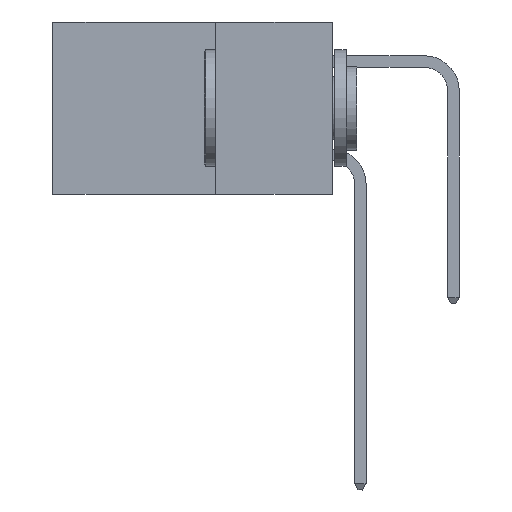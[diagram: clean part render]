
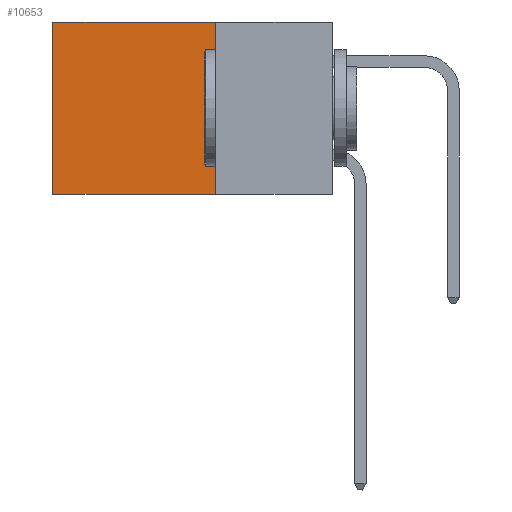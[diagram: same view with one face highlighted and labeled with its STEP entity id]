
A CAD part, left-side view. The second image highlights one B-rep face of the part: STEP entity #10653.
In plain terms, the highlighted planar face has unit normal (-1, 0, 0).
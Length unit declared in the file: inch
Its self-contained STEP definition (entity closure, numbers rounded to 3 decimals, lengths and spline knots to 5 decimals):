
#23 = DIRECTION ( 'NONE',  ( 0., 1., 0. ) ) ;
#202 = DIRECTION ( 'NONE',  ( 0., 1., 0. ) ) ;
#2963 = VERTEX_POINT ( 'NONE', #16725 ) ;
#3412 = CARTESIAN_POINT ( 'NONE',  ( 0.298, 0.25, 0. ) ) ;
#3432 = AXIS2_PLACEMENT_3D ( 'NONE', #3412, #16153, #6880 ) ;
#4799 = EDGE_LOOP ( 'NONE', ( #21293, #13506, #5982, #21306 ) ) ;
#5472 = VERTEX_POINT ( 'NONE', #6373 ) ;
#5982 = ORIENTED_EDGE ( 'NONE', *, *, #19559, .F. ) ;
#6373 = CARTESIAN_POINT ( 'NONE',  ( 0.298, 0.25, 0. ) ) ;
#6492 = VECTOR ( 'NONE', #22026, 39.37008 ) ;
#6506 = CARTESIAN_POINT ( 'NONE',  ( 0.298, 0.6, 0. ) ) ;
#6880 = DIRECTION ( 'NONE',  ( 0., 0., -1. ) ) ;
#7094 = CARTESIAN_POINT ( 'NONE',  ( 0.298, 0.25, 0. ) ) ;
#7460 = VERTEX_POINT ( 'NONE', #18580 ) ;
#9007 = EDGE_CURVE ( 'NONE', #17742, #2963, #20754, .T. ) ;
#10580 = PLANE ( 'NONE',  #3432 ) ;
#10653 = ADVANCED_FACE ( 'NONE', ( #21279 ), #10580, .F. ) ;
#10973 = LINE ( 'NONE', #19031, #15014 ) ;
#13506 = ORIENTED_EDGE ( 'NONE', *, *, #14311, .F. ) ;
#13612 = VECTOR ( 'NONE', #23, 39.37008 ) ;
#14311 = EDGE_CURVE ( 'NONE', #7460, #2963, #17060, .T. ) ;
#14772 = CARTESIAN_POINT ( 'NONE',  ( 0.298, 0.25, -0.37 ) ) ;
#14782 = VECTOR ( 'NONE', #19998, 39.37008 ) ;
#15014 = VECTOR ( 'NONE', #202, 39.37008 ) ;
#15074 = LINE ( 'NONE', #7094, #14782 ) ;
#16153 = DIRECTION ( 'NONE',  ( 1., 0., 0. ) ) ;
#16501 = CARTESIAN_POINT ( 'NONE',  ( 0.298, 0.6, 0. ) ) ;
#16725 = CARTESIAN_POINT ( 'NONE',  ( 0.298, 0.6, -0.37 ) ) ;
#17060 = LINE ( 'NONE', #14772, #13612 ) ;
#17742 = VERTEX_POINT ( 'NONE', #6506 ) ;
#18580 = CARTESIAN_POINT ( 'NONE',  ( 0.298, 0.25, -0.37 ) ) ;
#19031 = CARTESIAN_POINT ( 'NONE',  ( 0.298, 0.25, 0. ) ) ;
#19559 = EDGE_CURVE ( 'NONE', #5472, #7460, #15074, .T. ) ;
#19998 = DIRECTION ( 'NONE',  ( 0., 0., -1. ) ) ;
#20754 = LINE ( 'NONE', #16501, #6492 ) ;
#21279 = FACE_OUTER_BOUND ( 'NONE', #4799, .T. ) ;
#21289 = EDGE_CURVE ( 'NONE', #5472, #17742, #10973, .T. ) ;
#21293 = ORIENTED_EDGE ( 'NONE', *, *, #9007, .T. ) ;
#21306 = ORIENTED_EDGE ( 'NONE', *, *, #21289, .T. ) ;
#22026 = DIRECTION ( 'NONE',  ( 0., 0., -1. ) ) ;
